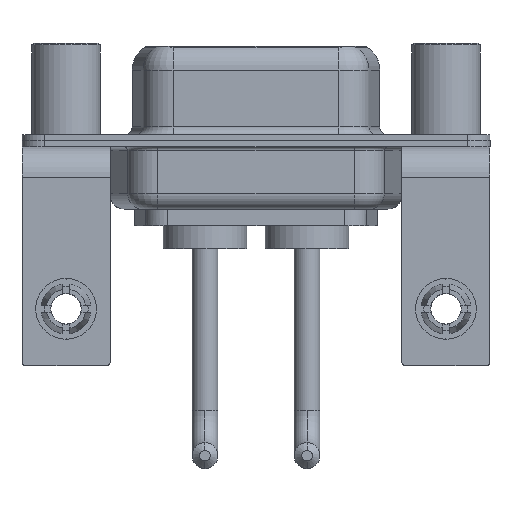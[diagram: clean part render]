
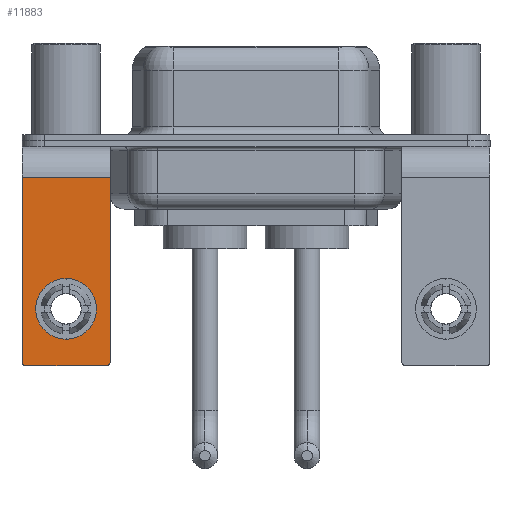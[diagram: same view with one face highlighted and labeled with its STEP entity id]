
A CAD part, front view. The second image highlights one B-rep face of the part: STEP entity #11883.
In plain terms, the highlighted planar face has unit normal (0, -1, 0).
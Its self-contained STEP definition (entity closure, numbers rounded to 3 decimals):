
#265 = VERTEX_POINT ( 'NONE', #12113 ) ;
#276 = DIRECTION ( 'NONE',  ( 0., 0., -1. ) ) ;
#563 = ORIENTED_EDGE ( 'NONE', *, *, #11052, .F. ) ;
#669 = CIRCLE ( 'NONE', #11588, 0.25 ) ;
#1076 = CARTESIAN_POINT ( 'NONE',  ( 2.9, -6.25, -14.55 ) ) ;
#1175 = VECTOR ( 'NONE', #6690, 1000. ) ;
#1335 = CARTESIAN_POINT ( 'NONE',  ( 2.65, -6.25, -14.8 ) ) ;
#1860 = CARTESIAN_POINT ( 'NONE',  ( 0., -6.25, -13.07 ) ) ;
#1934 = VERTEX_POINT ( 'NONE', #14451 ) ;
#2065 = LINE ( 'NONE', #3498, #5025 ) ;
#2071 = DIRECTION ( 'NONE',  ( 0., 0., 1. ) ) ;
#2193 = CARTESIAN_POINT ( 'NONE',  ( 2.9, -6.25, -2.4 ) ) ;
#2298 = DIRECTION ( 'NONE',  ( -1., 0., 0. ) ) ;
#2385 = CARTESIAN_POINT ( 'NONE',  ( 2.65, -6.25, -14.55 ) ) ;
#2476 = VECTOR ( 'NONE', #12877, 1000. ) ;
#2656 = ORIENTED_EDGE ( 'NONE', *, *, #7036, .T. ) ;
#3032 = EDGE_CURVE ( 'NONE', #12153, #4256, #12608, .T. ) ;
#3037 = CARTESIAN_POINT ( 'NONE',  ( -2.65, -6.25, -14.8 ) ) ;
#3498 = CARTESIAN_POINT ( 'NONE',  ( 2.9, -6.25, -14.8 ) ) ;
#3697 = EDGE_LOOP ( 'NONE', ( #3878, #9065, #4521, #11119, #563, #2656 ) ) ;
#3878 = ORIENTED_EDGE ( 'NONE', *, *, #8419, .T. ) ;
#3937 = DIRECTION ( 'NONE',  ( 0., 1., 0. ) ) ;
#4256 = VERTEX_POINT ( 'NONE', #6585 ) ;
#4521 = ORIENTED_EDGE ( 'NONE', *, *, #8565, .F. ) ;
#4599 = ORIENTED_EDGE ( 'NONE', *, *, #8023, .T. ) ;
#4615 = VERTEX_POINT ( 'NONE', #3037 ) ;
#5025 = VECTOR ( 'NONE', #2298, 1000. ) ;
#5204 = DIRECTION ( 'NONE',  ( 0., 1., 0. ) ) ;
#5769 = AXIS2_PLACEMENT_3D ( 'NONE', #5958, #5204, #8858 ) ;
#5958 = CARTESIAN_POINT ( 'NONE',  ( 0., -6.25, -11.07 ) ) ;
#6458 = VERTEX_POINT ( 'NONE', #9233 ) ;
#6537 = CARTESIAN_POINT ( 'NONE',  ( -2.9, -6.25, -2.4 ) ) ;
#6585 = CARTESIAN_POINT ( 'NONE',  ( 0., -6.25, -9.07 ) ) ;
#6690 = DIRECTION ( 'NONE',  ( -1., 0., 0. ) ) ;
#7036 = EDGE_CURVE ( 'NONE', #6458, #265, #9212, .T. ) ;
#7062 = DIRECTION ( 'NONE',  ( 0., 0., 1. ) ) ;
#7457 = CARTESIAN_POINT ( 'NONE',  ( -2.65, -6.25, -14.55 ) ) ;
#7802 = CIRCLE ( 'NONE', #11115, 2. ) ;
#7823 = EDGE_CURVE ( 'NONE', #1934, #4615, #669, .T. ) ;
#7873 = AXIS2_PLACEMENT_3D ( 'NONE', #2385, #12965, #2071 ) ;
#8023 = EDGE_CURVE ( 'NONE', #4256, #12153, #7802, .T. ) ;
#8243 = VERTEX_POINT ( 'NONE', #1076 ) ;
#8404 = FACE_OUTER_BOUND ( 'NONE', #3697, .T. ) ;
#8408 = DIRECTION ( 'NONE',  ( 0., -1., 0. ) ) ;
#8419 = EDGE_CURVE ( 'NONE', #265, #1934, #12797, .T. ) ;
#8565 = EDGE_CURVE ( 'NONE', #12757, #4615, #2065, .T. ) ;
#8858 = DIRECTION ( 'NONE',  ( 0., 0., 1. ) ) ;
#9065 = ORIENTED_EDGE ( 'NONE', *, *, #7823, .T. ) ;
#9212 = LINE ( 'NONE', #14067, #1175 ) ;
#9233 = CARTESIAN_POINT ( 'NONE',  ( 2.9, -6.25, -2.4 ) ) ;
#9744 = FACE_BOUND ( 'NONE', #10093, .T. ) ;
#9902 = VECTOR ( 'NONE', #276, 1000. ) ;
#10093 = EDGE_LOOP ( 'NONE', ( #13902, #4599 ) ) ;
#11052 = EDGE_CURVE ( 'NONE', #6458, #8243, #15261, .T. ) ;
#11115 = AXIS2_PLACEMENT_3D ( 'NONE', #14835, #3937, #11490 ) ;
#11119 = ORIENTED_EDGE ( 'NONE', *, *, #11290, .T. ) ;
#11290 = EDGE_CURVE ( 'NONE', #12757, #8243, #12666, .T. ) ;
#11490 = DIRECTION ( 'NONE',  ( 0., 0., 1. ) ) ;
#11588 = AXIS2_PLACEMENT_3D ( 'NONE', #7457, #8408, #12294 ) ;
#11883 = ADVANCED_FACE ( 'NONE', ( #9744, #8404 ), #12056, .F. ) ;
#12056 = PLANE ( 'NONE',  #15196 ) ;
#12113 = CARTESIAN_POINT ( 'NONE',  ( -2.9, -6.25, -2.4 ) ) ;
#12153 = VERTEX_POINT ( 'NONE', #1860 ) ;
#12294 = DIRECTION ( 'NONE',  ( 0., 0., 1. ) ) ;
#12357 = CARTESIAN_POINT ( 'NONE',  ( 2.9, -6.25, -2.4 ) ) ;
#12608 = CIRCLE ( 'NONE', #5769, 2. ) ;
#12666 = CIRCLE ( 'NONE', #7873, 0.25 ) ;
#12757 = VERTEX_POINT ( 'NONE', #1335 ) ;
#12797 = LINE ( 'NONE', #6537, #2476 ) ;
#12877 = DIRECTION ( 'NONE',  ( 0., 0., -1. ) ) ;
#12965 = DIRECTION ( 'NONE',  ( 0., -1., 0. ) ) ;
#13902 = ORIENTED_EDGE ( 'NONE', *, *, #3032, .T. ) ;
#14067 = CARTESIAN_POINT ( 'NONE',  ( 2.9, -6.25, -2.4 ) ) ;
#14451 = CARTESIAN_POINT ( 'NONE',  ( -2.9, -6.25, -14.55 ) ) ;
#14835 = CARTESIAN_POINT ( 'NONE',  ( 0., -6.25, -11.07 ) ) ;
#15196 = AXIS2_PLACEMENT_3D ( 'NONE', #2193, #15555, #7062 ) ;
#15261 = LINE ( 'NONE', #12357, #9902 ) ;
#15555 = DIRECTION ( 'NONE',  ( 0., 1., 0. ) ) ;
